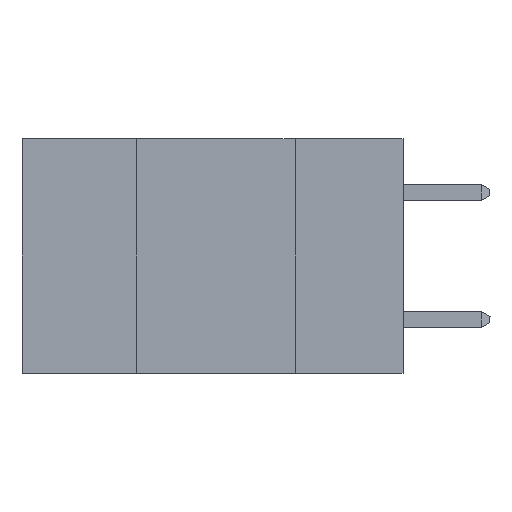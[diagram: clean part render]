
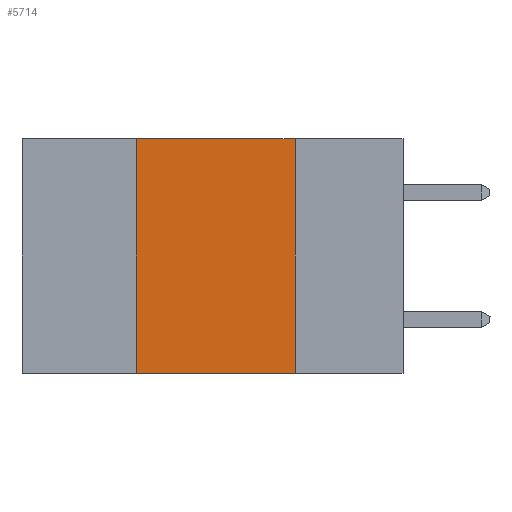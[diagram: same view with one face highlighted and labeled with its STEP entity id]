
A CAD part, left-side view. The second image highlights one B-rep face of the part: STEP entity #5714.
In plain terms, the highlighted planar face has unit normal (-1, 0, 0).
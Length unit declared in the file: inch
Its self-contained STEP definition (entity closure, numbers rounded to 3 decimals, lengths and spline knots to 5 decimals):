
#473 = ORIENTED_EDGE ( 'NONE', *, *, #12064, .T. ) ;
#1654 = EDGE_LOOP ( 'NONE', ( #9052, #15903, #18174, #473 ) ) ;
#1986 = EDGE_CURVE ( 'NONE', #14071, #4056, #4809, .T. ) ;
#2050 = DIRECTION ( 'NONE',  ( 0., 0., -1. ) ) ;
#2573 = LINE ( 'NONE', #11528, #13596 ) ;
#3661 = DIRECTION ( 'NONE',  ( 0., -1., 0. ) ) ;
#4056 = VERTEX_POINT ( 'NONE', #12691 ) ;
#4809 = LINE ( 'NONE', #5375, #20159 ) ;
#5375 = CARTESIAN_POINT ( 'NONE',  ( 0., 0.6, 0. ) ) ;
#5714 = ADVANCED_FACE ( 'NONE', ( #19509 ), #14779, .F. ) ;
#5906 = DIRECTION ( 'NONE',  ( 0., 0., 1. ) ) ;
#6699 = LINE ( 'NONE', #16634, #10486 ) ;
#6914 = CARTESIAN_POINT ( 'NONE',  ( 0., 0.17, -0.37 ) ) ;
#7022 = CARTESIAN_POINT ( 'NONE',  ( 0., 0.42, -0.37 ) ) ;
#9052 = ORIENTED_EDGE ( 'NONE', *, *, #9069, .F. ) ;
#9069 = EDGE_CURVE ( 'NONE', #4056, #20732, #2573, .T. ) ;
#9556 = LINE ( 'NONE', #18189, #17094 ) ;
#10160 = DIRECTION ( 'NONE',  ( 0., -1., 0. ) ) ;
#10486 = VECTOR ( 'NONE', #3661, 39.37008 ) ;
#11528 = CARTESIAN_POINT ( 'NONE',  ( 0., 0.17, 0. ) ) ;
#12064 = EDGE_CURVE ( 'NONE', #13088, #20732, #6699, .T. ) ;
#12691 = CARTESIAN_POINT ( 'NONE',  ( 0., 0.17, 0. ) ) ;
#13088 = VERTEX_POINT ( 'NONE', #7022 ) ;
#13408 = CARTESIAN_POINT ( 'NONE',  ( 0., 0.6, 0. ) ) ;
#13596 = VECTOR ( 'NONE', #19725, 39.37008 ) ;
#14071 = VERTEX_POINT ( 'NONE', #19407 ) ;
#14779 = PLANE ( 'NONE',  #15309 ) ;
#15309 = AXIS2_PLACEMENT_3D ( 'NONE', #13408, #16425, #2050 ) ;
#15903 = ORIENTED_EDGE ( 'NONE', *, *, #1986, .F. ) ;
#16361 = EDGE_CURVE ( 'NONE', #13088, #14071, #9556, .T. ) ;
#16425 = DIRECTION ( 'NONE',  ( 1., 0., 0. ) ) ;
#16634 = CARTESIAN_POINT ( 'NONE',  ( 0., 0.6, -0.37 ) ) ;
#17094 = VECTOR ( 'NONE', #5906, 39.37008 ) ;
#18174 = ORIENTED_EDGE ( 'NONE', *, *, #16361, .F. ) ;
#18189 = CARTESIAN_POINT ( 'NONE',  ( 0., 0.42, 0. ) ) ;
#19407 = CARTESIAN_POINT ( 'NONE',  ( 0., 0.42, 0. ) ) ;
#19509 = FACE_OUTER_BOUND ( 'NONE', #1654, .T. ) ;
#19725 = DIRECTION ( 'NONE',  ( 0., 0., -1. ) ) ;
#20159 = VECTOR ( 'NONE', #10160, 39.37008 ) ;
#20732 = VERTEX_POINT ( 'NONE', #6914 ) ;
